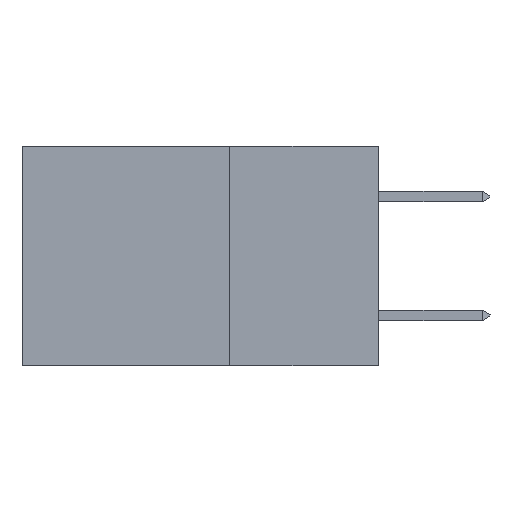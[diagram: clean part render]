
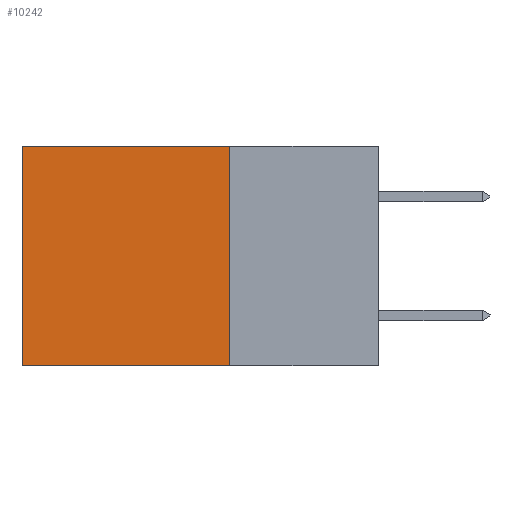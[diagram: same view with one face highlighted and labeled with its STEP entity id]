
A CAD part, left-side view. The second image highlights one B-rep face of the part: STEP entity #10242.
In plain terms, the highlighted planar face has unit normal (-1, 0, 0).
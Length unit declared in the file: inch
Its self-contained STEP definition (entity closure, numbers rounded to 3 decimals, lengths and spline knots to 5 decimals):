
#1664 = DIRECTION ( 'NONE',  ( 0., 1., 0. ) ) ;
#2474 = DIRECTION ( 'NONE',  ( 0., 0., -1. ) ) ;
#2582 = LINE ( 'NONE', #20861, #19774 ) ;
#7297 = EDGE_CURVE ( 'NONE', #21209, #16450, #8770, .T. ) ;
#7444 = FACE_OUTER_BOUND ( 'NONE', #8236, .T. ) ;
#7536 = DIRECTION ( 'NONE',  ( 1., 0., 0. ) ) ;
#8236 = EDGE_LOOP ( 'NONE', ( #18999, #9458, #11522, #15265 ) ) ;
#8770 = LINE ( 'NONE', #16690, #14484 ) ;
#8898 = CARTESIAN_POINT ( 'NONE',  ( 0.298, 0.6, 0. ) ) ;
#9458 = ORIENTED_EDGE ( 'NONE', *, *, #20359, .F. ) ;
#10242 = ADVANCED_FACE ( 'NONE', ( #7444 ), #15822, .F. ) ;
#11320 = VECTOR ( 'NONE', #14428, 39.37008 ) ;
#11522 = ORIENTED_EDGE ( 'NONE', *, *, #7297, .F. ) ;
#11574 = LINE ( 'NONE', #12681, #11320 ) ;
#12157 = LINE ( 'NONE', #18329, #17382 ) ;
#12681 = CARTESIAN_POINT ( 'NONE',  ( 0.298, 0.25, 0. ) ) ;
#13272 = CARTESIAN_POINT ( 'NONE',  ( 0.298, 0.25, 0. ) ) ;
#14275 = VERTEX_POINT ( 'NONE', #20738 ) ;
#14284 = CARTESIAN_POINT ( 'NONE',  ( 0.298, 0.25, 0. ) ) ;
#14363 = DIRECTION ( 'NONE',  ( 0., 0., -1. ) ) ;
#14428 = DIRECTION ( 'NONE',  ( 0., 1., 0. ) ) ;
#14484 = VECTOR ( 'NONE', #18206, 39.37008 ) ;
#14761 = AXIS2_PLACEMENT_3D ( 'NONE', #14284, #7536, #14363 ) ;
#15265 = ORIENTED_EDGE ( 'NONE', *, *, #20868, .T. ) ;
#15822 = PLANE ( 'NONE',  #14761 ) ;
#16450 = VERTEX_POINT ( 'NONE', #20219 ) ;
#16690 = CARTESIAN_POINT ( 'NONE',  ( 0.298, 0.25, 0. ) ) ;
#17201 = EDGE_CURVE ( 'NONE', #19559, #14275, #2582, .T. ) ;
#17382 = VECTOR ( 'NONE', #1664, 39.37008 ) ;
#18206 = DIRECTION ( 'NONE',  ( 0., 0., -1. ) ) ;
#18329 = CARTESIAN_POINT ( 'NONE',  ( 0.298, 0.25, -0.37 ) ) ;
#18999 = ORIENTED_EDGE ( 'NONE', *, *, #17201, .T. ) ;
#19559 = VERTEX_POINT ( 'NONE', #8898 ) ;
#19774 = VECTOR ( 'NONE', #2474, 39.37008 ) ;
#20219 = CARTESIAN_POINT ( 'NONE',  ( 0.298, 0.25, -0.37 ) ) ;
#20359 = EDGE_CURVE ( 'NONE', #16450, #14275, #12157, .T. ) ;
#20738 = CARTESIAN_POINT ( 'NONE',  ( 0.298, 0.6, -0.37 ) ) ;
#20861 = CARTESIAN_POINT ( 'NONE',  ( 0.298, 0.6, 0. ) ) ;
#20868 = EDGE_CURVE ( 'NONE', #21209, #19559, #11574, .T. ) ;
#21209 = VERTEX_POINT ( 'NONE', #13272 ) ;
